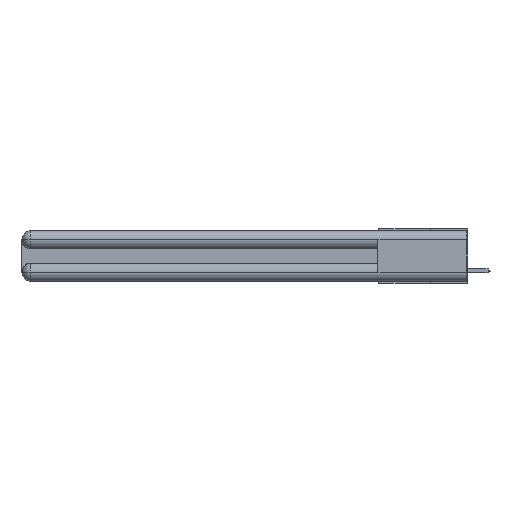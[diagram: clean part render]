
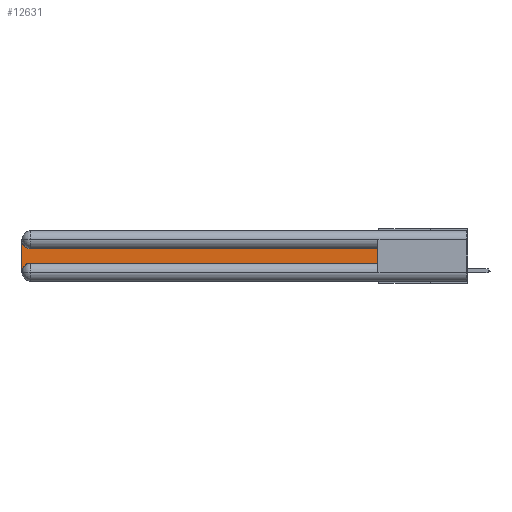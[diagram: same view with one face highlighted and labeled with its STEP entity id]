
A CAD part, left-side view. The second image highlights one B-rep face of the part: STEP entity #12631.
In plain terms, the highlighted planar face has unit normal (-1, 0, 0).
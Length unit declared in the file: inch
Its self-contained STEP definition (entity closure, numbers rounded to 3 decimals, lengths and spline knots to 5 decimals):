
#636 = CARTESIAN_POINT ( 'NONE',  ( 0.075, 3., -0.1225 ) ) ;
#886 = EDGE_LOOP ( 'NONE', ( #2673, #7482, #32100, #12794, #26233, #27530 ) ) ;
#1014 = CARTESIAN_POINT ( 'NONE',  ( 0.075, 0.6, -0.1225 ) ) ;
#1381 = CARTESIAN_POINT ( 'NONE',  ( 0.075, 0.6, -0.1225 ) ) ;
#1693 = CIRCLE ( 'NONE', #7623, 0.06 ) ;
#2673 = ORIENTED_EDGE ( 'NONE', *, *, #24520, .T. ) ;
#3540 = CARTESIAN_POINT ( 'NONE',  ( 0.075, 3., -0.2775 ) ) ;
#4156 = DIRECTION ( 'NONE',  ( 1., 0., 0. ) ) ;
#4234 = DIRECTION ( 'NONE',  ( 0., 0., -1. ) ) ;
#4242 = EDGE_CURVE ( 'NONE', #20021, #12574, #27471, .T. ) ;
#5451 = DIRECTION ( 'NONE',  ( 0., 0., -1. ) ) ;
#6965 = DIRECTION ( 'NONE',  ( 0., 0., -1. ) ) ;
#7482 = ORIENTED_EDGE ( 'NONE', *, *, #4242, .T. ) ;
#7623 = AXIS2_PLACEMENT_3D ( 'NONE', #21856, #22065, #6965 ) ;
#8514 = FACE_OUTER_BOUND ( 'NONE', #886, .T. ) ;
#8538 = VECTOR ( 'NONE', #4234, 39.37008 ) ;
#8929 = LINE ( 'NONE', #23854, #8538 ) ;
#9697 = CARTESIAN_POINT ( 'NONE',  ( 0.075, 3., -0.0625 ) ) ;
#10544 = VECTOR ( 'NONE', #28552, 39.37008 ) ;
#11372 = CARTESIAN_POINT ( 'NONE',  ( 0.075, 2.94, -0.2175 ) ) ;
#11649 = CARTESIAN_POINT ( 'NONE',  ( 0.075, 0.6, -0.2175 ) ) ;
#12051 = LINE ( 'NONE', #12454, #21517 ) ;
#12326 = EDGE_CURVE ( 'NONE', #12574, #23625, #8929, .T. ) ;
#12454 = CARTESIAN_POINT ( 'NONE',  ( 0.075, 0.6, -0.2175 ) ) ;
#12574 = VERTEX_POINT ( 'NONE', #9697 ) ;
#12631 = ADVANCED_FACE ( 'NONE', ( #8514 ), #20662, .F. ) ;
#12794 = ORIENTED_EDGE ( 'NONE', *, *, #18459, .T. ) ;
#13233 = VERTEX_POINT ( 'NONE', #1381 ) ;
#13283 = DIRECTION ( 'NONE',  ( 1., 0., 0. ) ) ;
#13624 = CARTESIAN_POINT ( 'NONE',  ( 0.075, 2.94, -0.0625 ) ) ;
#17301 = DIRECTION ( 'NONE',  ( 0., 0., 1. ) ) ;
#18393 = LINE ( 'NONE', #1014, #10544 ) ;
#18459 = EDGE_CURVE ( 'NONE', #23625, #32235, #1693, .T. ) ;
#18830 = VECTOR ( 'NONE', #24443, 39.37008 ) ;
#20021 = VERTEX_POINT ( 'NONE', #24211 ) ;
#20662 = PLANE ( 'NONE',  #22923 ) ;
#21517 = VECTOR ( 'NONE', #17301, 39.37008 ) ;
#21856 = CARTESIAN_POINT ( 'NONE',  ( 0.075, 2.94, -0.2775 ) ) ;
#22065 = DIRECTION ( 'NONE',  ( 1., 0., 0. ) ) ;
#22923 = AXIS2_PLACEMENT_3D ( 'NONE', #636, #13283, #5451 ) ;
#23625 = VERTEX_POINT ( 'NONE', #3540 ) ;
#23854 = CARTESIAN_POINT ( 'NONE',  ( 0.075, 3., -0.2175 ) ) ;
#24211 = CARTESIAN_POINT ( 'NONE',  ( 0.075, 2.94, -0.1225 ) ) ;
#24443 = DIRECTION ( 'NONE',  ( 0., -1., 0. ) ) ;
#24520 = EDGE_CURVE ( 'NONE', #13233, #20021, #18393, .T. ) ;
#24613 = EDGE_CURVE ( 'NONE', #32235, #25259, #27895, .T. ) ;
#25259 = VERTEX_POINT ( 'NONE', #27153 ) ;
#26233 = ORIENTED_EDGE ( 'NONE', *, *, #24613, .T. ) ;
#26777 = EDGE_CURVE ( 'NONE', #25259, #13233, #12051, .T. ) ;
#27153 = CARTESIAN_POINT ( 'NONE',  ( 0.075, 0.6, -0.2175 ) ) ;
#27471 = CIRCLE ( 'NONE', #29736, 0.06 ) ;
#27530 = ORIENTED_EDGE ( 'NONE', *, *, #26777, .T. ) ;
#27895 = LINE ( 'NONE', #11649, #18830 ) ;
#28552 = DIRECTION ( 'NONE',  ( 0., 1., 0. ) ) ;
#29736 = AXIS2_PLACEMENT_3D ( 'NONE', #13624, #4156, #31033 ) ;
#31033 = DIRECTION ( 'NONE',  ( 0., 0., -1. ) ) ;
#32100 = ORIENTED_EDGE ( 'NONE', *, *, #12326, .T. ) ;
#32235 = VERTEX_POINT ( 'NONE', #11372 ) ;
